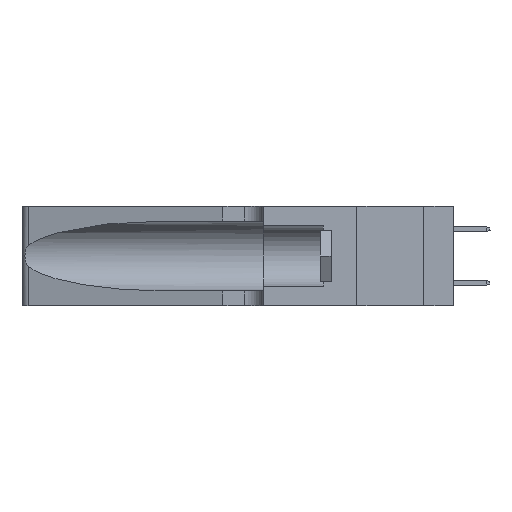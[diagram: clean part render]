
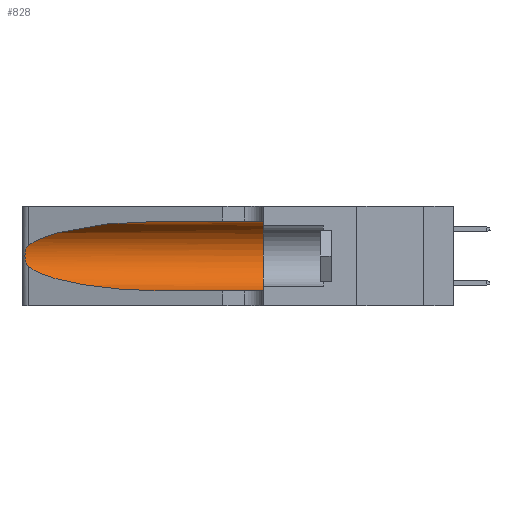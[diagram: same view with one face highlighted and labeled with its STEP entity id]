
A CAD part, left-side view. The second image highlights one B-rep face of the part: STEP entity #828.
In plain terms, the highlighted cylindrical face has radius 3.308 mm (diameter 6.617 mm), a partial arc.
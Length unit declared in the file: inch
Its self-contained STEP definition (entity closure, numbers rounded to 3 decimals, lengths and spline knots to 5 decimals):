
#828 = ADVANCED_FACE ( 'NONE', ( #4315 ), #12054, .F. ) ;
#833 = AXIS2_PLACEMENT_3D ( 'NONE', #30565, #26432, #35837 ) ;
#1024 = CARTESIAN_POINT ( 'NONE',  ( 0.26018, 1.23835, 0.19895 ) ) ;
#1852 = ORIENTED_EDGE ( 'NONE', *, *, #28362, .F. ) ;
#1962 = CARTESIAN_POINT ( 'NONE',  ( 0.1305, 1.61858, 0.31525 ) ) ;
#3118 = CARTESIAN_POINT ( 'NONE',  ( 0.18966, 0.96281, 0.05475 ) ) ;
#3380 = EDGE_CURVE ( 'NONE', #29684, #27373, #12122, .T. ) ;
#3689 = DIRECTION ( 'NONE',  ( 0., -1., 0. ) ) ;
#4315 = FACE_OUTER_BOUND ( 'NONE', #23330, .T. ) ;
#4495 = CARTESIAN_POINT ( 'NONE',  ( 0.2373, 1.15595, 0.28018 ) ) ;
#6566 = CARTESIAN_POINT ( 'NONE',  ( 0.1305, 1.61858, 0.05475 ) ) ;
#6975 = DIRECTION ( 'NONE',  ( 0., 0., 1. ) ) ;
#8063 = EDGE_CURVE ( 'NONE', #22272, #32318, #28006, .T. ) ;
#8404 = CARTESIAN_POINT ( 'NONE',  ( 0.25789, 1.23486, 0.15765 ) ) ;
#9460 = CARTESIAN_POINT ( 'NONE',  ( 0.25487, 1.22718, 0.14631 ) ) ;
#9467 = ORIENTED_EDGE ( 'NONE', *, *, #11545, .T. ) ;
#11545 = EDGE_CURVE ( 'NONE', #32318, #36826, #20942, .T. ) ;
#11686 = ORIENTED_EDGE ( 'NONE', *, *, #8063, .T. ) ;
#12028 = CARTESIAN_POINT ( 'NONE',  ( 0.1305, 0.72297, 0.05475 ) ) ;
#12054 = CYLINDRICAL_SURFACE ( 'NONE', #833, 0.13025 ) ;
#12122 =( BOUNDED_CURVE ( )  B_SPLINE_CURVE ( 3, ( #22681, #31514, #4495, #19267 ),
 .UNSPECIFIED., .F., .T. ) 
 B_SPLINE_CURVE_WITH_KNOTS ( ( 4, 4 ),
 ( 1.5708, 2.84003 ),
 .UNSPECIFIED. ) 
 CURVE ( )  GEOMETRIC_REPRESENTATION_ITEM ( )  RATIONAL_B_SPLINE_CURVE ( ( 1., 0.87, 0.87, 1. ) ) 
 REPRESENTATION_ITEM ( '' )  );
#12612 = EDGE_CURVE ( 'NONE', #29684, #35363, #27671, .T. ) ;
#12720 = CARTESIAN_POINT ( 'NONE',  ( 0.26017, 1.23833, 0.17102 ) ) ;
#13110 = DIRECTION ( 'NONE',  ( 0., -1., 0. ) ) ;
#14338 = CARTESIAN_POINT ( 'NONE',  ( 0.25854, 1.2359, 0.20912 ) ) ;
#14832 = CARTESIAN_POINT ( 'NONE',  ( 0.1305, 0.72297, 0.05475 ) ) ;
#15611 = CARTESIAN_POINT ( 'NONE',  ( 0.25787, 1.23484, 0.2124 ) ) ;
#16168 = ORIENTED_EDGE ( 'NONE', *, *, #12612, .F. ) ;
#16460 = AXIS2_PLACEMENT_3D ( 'NONE', #36337, #21734, #6975 ) ;
#17022 = ORIENTED_EDGE ( 'NONE', *, *, #30571, .T. ) ;
#17635 = CARTESIAN_POINT ( 'NONE',  ( 0.1305, 0.35, 0.05475 ) ) ;
#18384 = VECTOR ( 'NONE', #13110, 39.37008 ) ;
#19267 = CARTESIAN_POINT ( 'NONE',  ( 0.25487, 1.22718, 0.22369 ) ) ;
#20104 = CARTESIAN_POINT ( 'NONE',  ( 0.25555, 1.22993, 0.14849 ) ) ;
#20286 = CARTESIAN_POINT ( 'NONE',  ( 0.25555, 1.22994, 0.2215 ) ) ;
#20942 = LINE ( 'NONE', #6566, #37425 ) ;
#21694 = CARTESIAN_POINT ( 'NONE',  ( 0.25487, 1.22718, 0.14631 ) ) ;
#21734 = DIRECTION ( 'NONE',  ( 0., 1., 0. ) ) ;
#22272 = VERTEX_POINT ( 'NONE', #21694 ) ;
#22681 = CARTESIAN_POINT ( 'NONE',  ( 0.1305, 0.72297, 0.31525 ) ) ;
#23213 = CIRCLE ( 'NONE', #16460, 0.13025 ) ;
#23330 = EDGE_LOOP ( 'NONE', ( #34496, #17022, #11686, #9467, #1852, #16168 ) ) ;
#24403 = CARTESIAN_POINT ( 'NONE',  ( 0.25856, 1.23593, 0.16098 ) ) ;
#26028 = CARTESIAN_POINT ( 'NONE',  ( 0.25639, 1.23186, 0.15144 ) ) ;
#26213 = CARTESIAN_POINT ( 'NONE',  ( 0.26075, 1.23896, 0.178 ) ) ;
#26432 = DIRECTION ( 'NONE',  ( 0., -1., 0. ) ) ;
#26725 = B_SPLINE_CURVE_WITH_KNOTS ( 'NONE', 3,
 ( #35962, #20286, #30175, #15611, #14338, #1024, #27290, #26213, #12720, #24403, #8404, #26028, #20104, #31782 ),
 .UNSPECIFIED., .F., .F.,
 ( 4, 2, 2, 2, 2, 2, 4 ),
 ( 0., 0.00027, 0.00053, 0.00107, 0.0016, 0.00187, 0.00214 ),
 .UNSPECIFIED. ) ;
#27290 = CARTESIAN_POINT ( 'NONE',  ( 0.26075, 1.23896, 0.19203 ) ) ;
#27373 = VERTEX_POINT ( 'NONE', #34021 ) ;
#27671 = LINE ( 'NONE', #1962, #18384 ) ;
#28006 =( BOUNDED_CURVE ( )  B_SPLINE_CURVE ( 3, ( #9460, #32462, #3118, #14832 ),
 .UNSPECIFIED., .F., .T. ) 
 B_SPLINE_CURVE_WITH_KNOTS ( ( 4, 4 ),
 ( 3.44316, 4.71239 ),
 .UNSPECIFIED. ) 
 CURVE ( )  GEOMETRIC_REPRESENTATION_ITEM ( )  RATIONAL_B_SPLINE_CURVE ( ( 1., 0.87, 0.87, 1. ) ) 
 REPRESENTATION_ITEM ( '' )  );
#28362 = EDGE_CURVE ( 'NONE', #35363, #36826, #23213, .T. ) ;
#28825 = CARTESIAN_POINT ( 'NONE',  ( 0.1305, 0.72297, 0.31525 ) ) ;
#29684 = VERTEX_POINT ( 'NONE', #28825 ) ;
#30175 = CARTESIAN_POINT ( 'NONE',  ( 0.25639, 1.23184, 0.21858 ) ) ;
#30565 = CARTESIAN_POINT ( 'NONE',  ( 0.1305, 1.61858, 0.185 ) ) ;
#30571 = EDGE_CURVE ( 'NONE', #27373, #22272, #26725, .T. ) ;
#31514 = CARTESIAN_POINT ( 'NONE',  ( 0.18966, 0.96281, 0.31525 ) ) ;
#31782 = CARTESIAN_POINT ( 'NONE',  ( 0.25487, 1.22718, 0.14631 ) ) ;
#32318 = VERTEX_POINT ( 'NONE', #12028 ) ;
#32462 = CARTESIAN_POINT ( 'NONE',  ( 0.2373, 1.15595, 0.08982 ) ) ;
#34021 = CARTESIAN_POINT ( 'NONE',  ( 0.25487, 1.22718, 0.22369 ) ) ;
#34496 = ORIENTED_EDGE ( 'NONE', *, *, #3380, .T. ) ;
#35363 = VERTEX_POINT ( 'NONE', #36902 ) ;
#35837 = DIRECTION ( 'NONE',  ( 0., 0., -1. ) ) ;
#35962 = CARTESIAN_POINT ( 'NONE',  ( 0.25487, 1.22718, 0.22369 ) ) ;
#36337 = CARTESIAN_POINT ( 'NONE',  ( 0.1305, 0.35, 0.185 ) ) ;
#36826 = VERTEX_POINT ( 'NONE', #17635 ) ;
#36902 = CARTESIAN_POINT ( 'NONE',  ( 0.1305, 0.35, 0.31525 ) ) ;
#37425 = VECTOR ( 'NONE', #3689, 39.37008 ) ;
